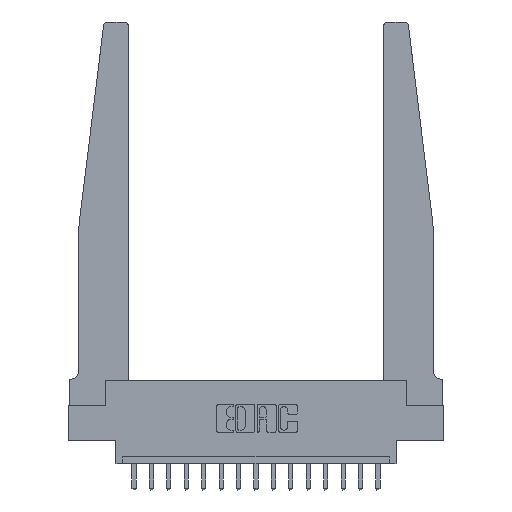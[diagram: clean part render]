
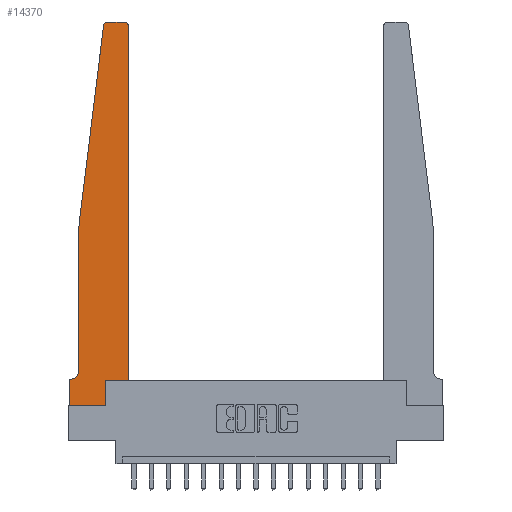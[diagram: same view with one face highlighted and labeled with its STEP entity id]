
A CAD part, top view. The second image highlights one B-rep face of the part: STEP entity #14370.
In plain terms, the highlighted planar face has unit normal (0, 0, 1).
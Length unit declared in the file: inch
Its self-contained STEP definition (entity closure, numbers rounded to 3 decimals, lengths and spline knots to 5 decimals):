
#153 = CARTESIAN_POINT ( 'NONE',  ( 0.2605, 0., 0.37 ) ) ;
#285 = DIRECTION ( 'NONE',  ( 0., 1., 0. ) ) ;
#416 = VECTOR ( 'NONE', #2916, 39.37008 ) ;
#616 = EDGE_CURVE ( 'NONE', #3354, #9840, #3067, .T. ) ;
#1185 = ORIENTED_EDGE ( 'NONE', *, *, #17005, .T. ) ;
#1705 = ORIENTED_EDGE ( 'NONE', *, *, #6722, .T. ) ;
#1869 = DIRECTION ( 'NONE',  ( 1., 0., 0. ) ) ;
#2043 = CARTESIAN_POINT ( 'NONE',  ( 0.015, 0.1875, 0.37 ) ) ;
#2113 = VECTOR ( 'NONE', #285, 39.37008 ) ;
#2139 = DIRECTION ( 'NONE',  ( 0., 0., 1. ) ) ;
#2843 = CARTESIAN_POINT ( 'NONE',  ( 0.24675, 2.72367, 0.37 ) ) ;
#2916 = DIRECTION ( 'NONE',  ( 0., 1., 0. ) ) ;
#3056 = CARTESIAN_POINT ( 'NONE',  ( 0.395, 2.75, 0.37 ) ) ;
#3067 = LINE ( 'NONE', #4193, #17358 ) ;
#3114 = VERTEX_POINT ( 'NONE', #12165 ) ;
#3213 = CARTESIAN_POINT ( 'NONE',  ( 0.2605, 0.18, 0.37 ) ) ;
#3354 = VERTEX_POINT ( 'NONE', #16710 ) ;
#3579 = CARTESIAN_POINT ( 'NONE',  ( 0., 0.1875, 0.37 ) ) ;
#3598 = VERTEX_POINT ( 'NONE', #2843 ) ;
#4183 = EDGE_CURVE ( 'NONE', #13080, #3354, #13989, .T. ) ;
#4193 = CARTESIAN_POINT ( 'NONE',  ( 0., 0., 0.37 ) ) ;
#4292 = LINE ( 'NONE', #3213, #2113 ) ;
#4397 = EDGE_CURVE ( 'NONE', #6252, #8538, #11377, .T. ) ;
#4571 = CIRCLE ( 'NONE', #15890, 0.03 ) ;
#4850 = VECTOR ( 'NONE', #4947, 39.37008 ) ;
#4866 = DIRECTION ( 'NONE',  ( 1., 0., 0. ) ) ;
#4947 = DIRECTION ( 'NONE',  ( 0., -1., 0. ) ) ;
#5237 = DIRECTION ( 'NONE',  ( -1., 0., 0. ) ) ;
#5259 = CARTESIAN_POINT ( 'NONE',  ( 0.425, 0.18, 0.37 ) ) ;
#6252 = VERTEX_POINT ( 'NONE', #9472 ) ;
#6318 = DIRECTION ( 'NONE',  ( -1., 0., 0. ) ) ;
#6668 = AXIS2_PLACEMENT_3D ( 'NONE', #12061, #13360, #10631 ) ;
#6722 = EDGE_CURVE ( 'NONE', #3598, #7463, #9817, .T. ) ;
#6807 = CARTESIAN_POINT ( 'NONE',  ( 0., 0.1875, 0.37 ) ) ;
#6878 = DIRECTION ( 'NONE',  ( 1., 0., 0. ) ) ;
#7463 = VERTEX_POINT ( 'NONE', #8054 ) ;
#7672 = LINE ( 'NONE', #10896, #7876 ) ;
#7876 = VECTOR ( 'NONE', #5237, 39.37008 ) ;
#7925 = ORIENTED_EDGE ( 'NONE', *, *, #12434, .T. ) ;
#8028 = CARTESIAN_POINT ( 'NONE',  ( 0.425, 0.18, 0.37 ) ) ;
#8054 = CARTESIAN_POINT ( 'NONE',  ( 0.065, 1.25, 0.37 ) ) ;
#8100 = CARTESIAN_POINT ( 'NONE',  ( 0.2605, 0.18, 0.37 ) ) ;
#8140 = ORIENTED_EDGE ( 'NONE', *, *, #12274, .T. ) ;
#8160 = EDGE_CURVE ( 'NONE', #3114, #14172, #11753, .T. ) ;
#8268 = FACE_OUTER_BOUND ( 'NONE', #11424, .T. ) ;
#8538 = VERTEX_POINT ( 'NONE', #2043 ) ;
#8574 = VECTOR ( 'NONE', #6318, 39.37008 ) ;
#9021 = CARTESIAN_POINT ( 'NONE',  ( 0.065, 1.25, 0.37 ) ) ;
#9047 = VECTOR ( 'NONE', #6878, 39.37008 ) ;
#9121 = LINE ( 'NONE', #9021, #4850 ) ;
#9472 = CARTESIAN_POINT ( 'NONE',  ( 0.065, 0.2375, 0.37 ) ) ;
#9817 = LINE ( 'NONE', #13669, #13487 ) ;
#9840 = VERTEX_POINT ( 'NONE', #153 ) ;
#10160 = DIRECTION ( 'NONE',  ( 0., -1., 0. ) ) ;
#10269 = CARTESIAN_POINT ( 'NONE',  ( 0.25, 2.75, 0.37 ) ) ;
#10442 = ORIENTED_EDGE ( 'NONE', *, *, #4397, .T. ) ;
#10631 = DIRECTION ( 'NONE',  ( 1., 0., 0. ) ) ;
#10695 = CARTESIAN_POINT ( 'NONE',  ( 0.27653, 2.75, 0.37 ) ) ;
#10734 = ORIENTED_EDGE ( 'NONE', *, *, #12189, .T. ) ;
#10835 = DIRECTION ( 'NONE',  ( 0., 0., -1. ) ) ;
#10896 = CARTESIAN_POINT ( 'NONE',  ( 0.065, 0.1875, 0.37 ) ) ;
#10933 = LINE ( 'NONE', #10269, #8574 ) ;
#11110 = DIRECTION ( 'NONE',  ( 1., 0., 0. ) ) ;
#11344 = DIRECTION ( 'NONE',  ( 0., 0., 1. ) ) ;
#11377 = CIRCLE ( 'NONE', #12633, 0.05 ) ;
#11424 = EDGE_LOOP ( 'NONE', ( #7925, #1185, #1705, #13352, #10442, #14844, #12609, #17185, #16243, #10734, #8140, #13446 ) ) ;
#11753 = CIRCLE ( 'NONE', #6668, 0.03 ) ;
#11898 = EDGE_CURVE ( 'NONE', #9840, #14859, #4292, .T. ) ;
#12061 = CARTESIAN_POINT ( 'NONE',  ( 0.395, 2.72, 0.37 ) ) ;
#12165 = CARTESIAN_POINT ( 'NONE',  ( 0.425, 2.72, 0.37 ) ) ;
#12189 = EDGE_CURVE ( 'NONE', #14859, #16789, #16872, .T. ) ;
#12274 = EDGE_CURVE ( 'NONE', #16789, #3114, #16044, .T. ) ;
#12323 = DIRECTION ( 'NONE',  ( -1., 0., 0. ) ) ;
#12434 = EDGE_CURVE ( 'NONE', #14172, #14886, #10933, .T. ) ;
#12518 = VECTOR ( 'NONE', #10160, 39.37008 ) ;
#12609 = ORIENTED_EDGE ( 'NONE', *, *, #4183, .T. ) ;
#12633 = AXIS2_PLACEMENT_3D ( 'NONE', #13632, #10835, #12323 ) ;
#13080 = VERTEX_POINT ( 'NONE', #6807 ) ;
#13352 = ORIENTED_EDGE ( 'NONE', *, *, #14747, .T. ) ;
#13360 = DIRECTION ( 'NONE',  ( 0., 0., 1. ) ) ;
#13446 = ORIENTED_EDGE ( 'NONE', *, *, #8160, .T. ) ;
#13466 = EDGE_CURVE ( 'NONE', #8538, #13080, #7672, .T. ) ;
#13487 = VECTOR ( 'NONE', #13789, 39.37008 ) ;
#13632 = CARTESIAN_POINT ( 'NONE',  ( 0.015, 0.2375, 0.37 ) ) ;
#13655 = AXIS2_PLACEMENT_3D ( 'NONE', #3579, #2139, #4866 ) ;
#13669 = CARTESIAN_POINT ( 'NONE',  ( 0.065, 1.25, 0.37 ) ) ;
#13789 = DIRECTION ( 'NONE',  ( -0.122, -0.992, 0. ) ) ;
#13989 = LINE ( 'NONE', #14249, #12518 ) ;
#14172 = VERTEX_POINT ( 'NONE', #3056 ) ;
#14249 = CARTESIAN_POINT ( 'NONE',  ( 0., 0., 0.37 ) ) ;
#14370 = ADVANCED_FACE ( 'NONE', ( #8268 ), #15969, .T. ) ;
#14747 = EDGE_CURVE ( 'NONE', #7463, #6252, #9121, .T. ) ;
#14844 = ORIENTED_EDGE ( 'NONE', *, *, #13466, .T. ) ;
#14859 = VERTEX_POINT ( 'NONE', #8100 ) ;
#14886 = VERTEX_POINT ( 'NONE', #10695 ) ;
#15354 = CARTESIAN_POINT ( 'NONE',  ( 0.27653, 2.72, 0.37 ) ) ;
#15890 = AXIS2_PLACEMENT_3D ( 'NONE', #15354, #11344, #1869 ) ;
#15969 = PLANE ( 'NONE',  #13655 ) ;
#16044 = LINE ( 'NONE', #5259, #416 ) ;
#16243 = ORIENTED_EDGE ( 'NONE', *, *, #11898, .T. ) ;
#16304 = CARTESIAN_POINT ( 'NONE',  ( 0.425, 0.18, 0.37 ) ) ;
#16710 = CARTESIAN_POINT ( 'NONE',  ( 0., 0., 0.37 ) ) ;
#16789 = VERTEX_POINT ( 'NONE', #16304 ) ;
#16872 = LINE ( 'NONE', #8028, #9047 ) ;
#17005 = EDGE_CURVE ( 'NONE', #14886, #3598, #4571, .T. ) ;
#17185 = ORIENTED_EDGE ( 'NONE', *, *, #616, .T. ) ;
#17358 = VECTOR ( 'NONE', #11110, 39.37008 ) ;
